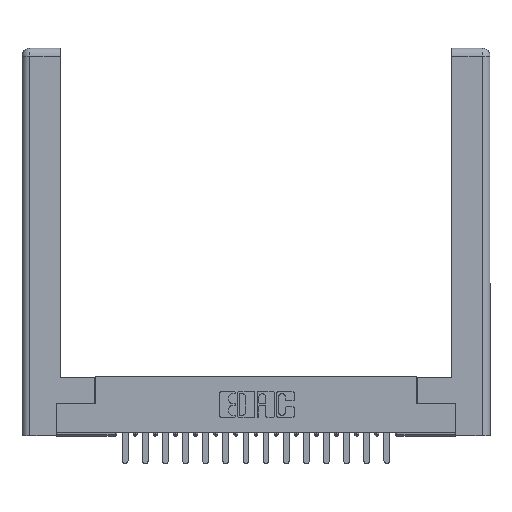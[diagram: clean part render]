
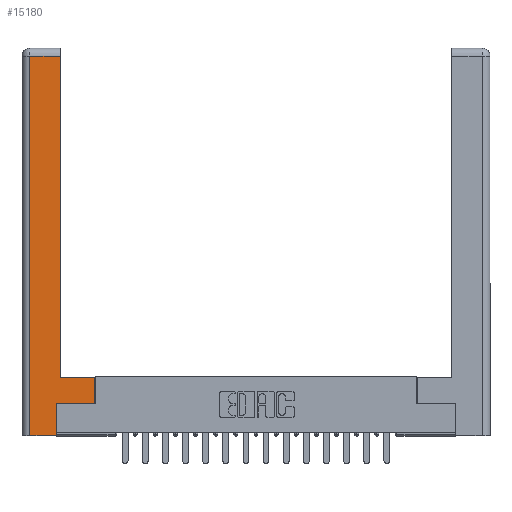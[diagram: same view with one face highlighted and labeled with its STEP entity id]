
A CAD part, top view. The second image highlights one B-rep face of the part: STEP entity #15180.
In plain terms, the highlighted planar face has unit normal (0, 0, 1).
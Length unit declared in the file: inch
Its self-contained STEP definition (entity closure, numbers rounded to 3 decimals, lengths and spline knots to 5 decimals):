
#52 = LINE ( 'NONE', #1764, #15338 ) ;
#274 = CARTESIAN_POINT ( 'NONE',  ( 0.565, 0.45, 0. ) ) ;
#388 = CARTESIAN_POINT ( 'NONE',  ( 0.295, 2.94, 0. ) ) ;
#532 = VECTOR ( 'NONE', #11892, 39.37008 ) ;
#732 = CARTESIAN_POINT ( 'NONE',  ( 0.0615, 0., 0. ) ) ;
#749 = ORIENTED_EDGE ( 'NONE', *, *, #10932, .T. ) ;
#1098 = EDGE_LOOP ( 'NONE', ( #9433, #8915, #749, #2045, #18923, #10995, #4748, #13373 ) ) ;
#1137 = LINE ( 'NONE', #10049, #16710 ) ;
#1153 = LINE ( 'NONE', #2346, #12612 ) ;
#1764 = CARTESIAN_POINT ( 'NONE',  ( 0.0615, 0., 0. ) ) ;
#1802 = EDGE_CURVE ( 'NONE', #16913, #9173, #1137, .T. ) ;
#2045 = ORIENTED_EDGE ( 'NONE', *, *, #1802, .T. ) ;
#2229 = DIRECTION ( 'NONE',  ( 0., 0., -1. ) ) ;
#2301 = LINE ( 'NONE', #16348, #7409 ) ;
#2346 = CARTESIAN_POINT ( 'NONE',  ( 0.265, 0.245, 0. ) ) ;
#2629 = VERTEX_POINT ( 'NONE', #18137 ) ;
#2933 = DIRECTION ( 'NONE',  ( -1., 0., 0. ) ) ;
#3634 = AXIS2_PLACEMENT_3D ( 'NONE', #5408, #2229, #10382 ) ;
#4748 = ORIENTED_EDGE ( 'NONE', *, *, #20210, .T. ) ;
#5408 = CARTESIAN_POINT ( 'NONE',  ( 0., 0., 0. ) ) ;
#5726 = DIRECTION ( 'NONE',  ( 0., 1., 0. ) ) ;
#6079 = VECTOR ( 'NONE', #14813, 39.37008 ) ;
#7409 = VECTOR ( 'NONE', #15756, 39.37008 ) ;
#7429 = VERTEX_POINT ( 'NONE', #19364 ) ;
#7901 = VERTEX_POINT ( 'NONE', #15191 ) ;
#7984 = CARTESIAN_POINT ( 'NONE',  ( 0.295, 0.45, 0. ) ) ;
#8915 = ORIENTED_EDGE ( 'NONE', *, *, #17290, .T. ) ;
#8945 = EDGE_CURVE ( 'NONE', #10632, #2629, #12576, .T. ) ;
#8948 = EDGE_CURVE ( 'NONE', #7901, #11700, #15393, .T. ) ;
#9173 = VERTEX_POINT ( 'NONE', #18692 ) ;
#9433 = ORIENTED_EDGE ( 'NONE', *, *, #17748, .T. ) ;
#9672 = CARTESIAN_POINT ( 'NONE',  ( 0.565, 0.245, 0. ) ) ;
#9840 = DIRECTION ( 'NONE',  ( 1., 0., 0. ) ) ;
#10049 = CARTESIAN_POINT ( 'NONE',  ( 0.265, 0., 0. ) ) ;
#10382 = DIRECTION ( 'NONE',  ( -1., 0., 0. ) ) ;
#10632 = VERTEX_POINT ( 'NONE', #17477 ) ;
#10932 = EDGE_CURVE ( 'NONE', #7429, #16913, #52, .T. ) ;
#10995 = ORIENTED_EDGE ( 'NONE', *, *, #8945, .T. ) ;
#11016 = CARTESIAN_POINT ( 'NONE',  ( 0.295, 0.45, 0. ) ) ;
#11021 = VECTOR ( 'NONE', #2933, 39.37008 ) ;
#11577 = VECTOR ( 'NONE', #17521, 39.37008 ) ;
#11700 = VERTEX_POINT ( 'NONE', #7984 ) ;
#11892 = DIRECTION ( 'NONE',  ( -1., 0., 0. ) ) ;
#12576 = LINE ( 'NONE', #9672, #11577 ) ;
#12612 = VECTOR ( 'NONE', #5726, 39.37008 ) ;
#13373 = ORIENTED_EDGE ( 'NONE', *, *, #8948, .T. ) ;
#13842 = EDGE_CURVE ( 'NONE', #9173, #10632, #1153, .T. ) ;
#14813 = DIRECTION ( 'NONE',  ( 0., 1., 0. ) ) ;
#15180 = ADVANCED_FACE ( 'NONE', ( #19223 ), #20957, .F. ) ;
#15191 = CARTESIAN_POINT ( 'NONE',  ( 0.565, 0.45, 0. ) ) ;
#15338 = VECTOR ( 'NONE', #18119, 39.37008 ) ;
#15393 = LINE ( 'NONE', #11016, #11021 ) ;
#15576 = LINE ( 'NONE', #20051, #532 ) ;
#15708 = VERTEX_POINT ( 'NONE', #388 ) ;
#15756 = DIRECTION ( 'NONE',  ( 0., 1., 0. ) ) ;
#16348 = CARTESIAN_POINT ( 'NONE',  ( 0.295, 3., 0. ) ) ;
#16710 = VECTOR ( 'NONE', #9840, 39.37008 ) ;
#16913 = VERTEX_POINT ( 'NONE', #732 ) ;
#17290 = EDGE_CURVE ( 'NONE', #15708, #7429, #15576, .T. ) ;
#17477 = CARTESIAN_POINT ( 'NONE',  ( 0.265, 0.245, 0. ) ) ;
#17521 = DIRECTION ( 'NONE',  ( 1., 0., 0. ) ) ;
#17748 = EDGE_CURVE ( 'NONE', #11700, #15708, #2301, .T. ) ;
#17754 = LINE ( 'NONE', #274, #6079 ) ;
#18119 = DIRECTION ( 'NONE',  ( 0., -1., 0. ) ) ;
#18137 = CARTESIAN_POINT ( 'NONE',  ( 0.565, 0.245, 0. ) ) ;
#18692 = CARTESIAN_POINT ( 'NONE',  ( 0.265, 0., 0. ) ) ;
#18923 = ORIENTED_EDGE ( 'NONE', *, *, #13842, .T. ) ;
#19223 = FACE_OUTER_BOUND ( 'NONE', #1098, .T. ) ;
#19364 = CARTESIAN_POINT ( 'NONE',  ( 0.0615, 2.94, 0. ) ) ;
#20051 = CARTESIAN_POINT ( 'NONE',  ( 0.0615, 2.94, 0. ) ) ;
#20210 = EDGE_CURVE ( 'NONE', #2629, #7901, #17754, .T. ) ;
#20957 = PLANE ( 'NONE',  #3634 ) ;
